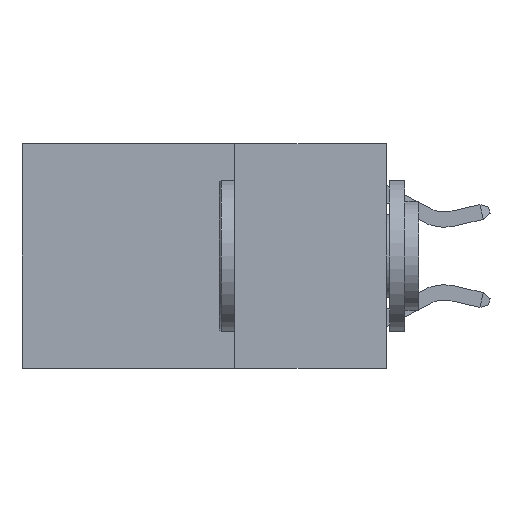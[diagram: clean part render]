
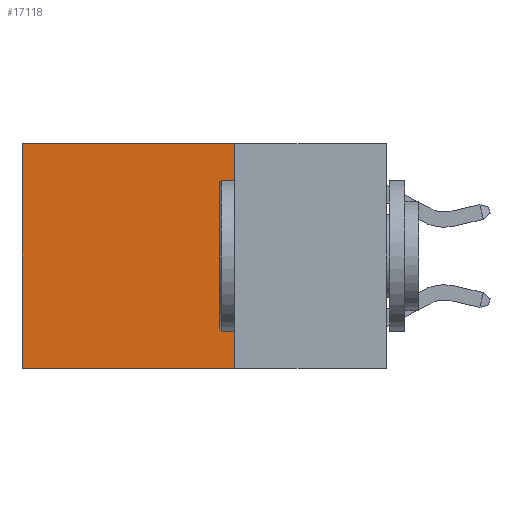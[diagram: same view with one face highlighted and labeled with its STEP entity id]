
A CAD part, left-side view. The second image highlights one B-rep face of the part: STEP entity #17118.
In plain terms, the highlighted planar face has unit normal (-1, 0, 0).
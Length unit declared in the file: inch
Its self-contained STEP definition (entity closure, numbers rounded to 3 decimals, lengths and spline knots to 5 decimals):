
#227 = FACE_OUTER_BOUND ( 'NONE', #14851, .T. ) ;
#1651 = CARTESIAN_POINT ( 'NONE',  ( 0.2625, 0.25, -0.37 ) ) ;
#2947 = CARTESIAN_POINT ( 'NONE',  ( 0.2625, 0.25, 0. ) ) ;
#3450 = EDGE_CURVE ( 'NONE', #28024, #12084, #20309, .T. ) ;
#3762 = CARTESIAN_POINT ( 'NONE',  ( 0.2625, 0.25, 0. ) ) ;
#4168 = DIRECTION ( 'NONE',  ( 0., 0., -1. ) ) ;
#4208 = DIRECTION ( 'NONE',  ( 0., 1., 0. ) ) ;
#4319 = LINE ( 'NONE', #11555, #26638 ) ;
#5220 = PLANE ( 'NONE',  #27787 ) ;
#6263 = EDGE_CURVE ( 'NONE', #12767, #10759, #6790, .T. ) ;
#6790 = LINE ( 'NONE', #1651, #8240 ) ;
#7896 = CARTESIAN_POINT ( 'NONE',  ( 0.2625, 0.6, -0.37 ) ) ;
#8240 = VECTOR ( 'NONE', #22434, 39.37008 ) ;
#9459 = DIRECTION ( 'NONE',  ( 1., 0., 0. ) ) ;
#9607 = DIRECTION ( 'NONE',  ( 0., 0., -1. ) ) ;
#10759 = VERTEX_POINT ( 'NONE', #7896 ) ;
#10929 = VECTOR ( 'NONE', #4208, 39.37008 ) ;
#11555 = CARTESIAN_POINT ( 'NONE',  ( 0.2625, 0.6, 0. ) ) ;
#12084 = VERTEX_POINT ( 'NONE', #19352 ) ;
#12743 = CARTESIAN_POINT ( 'NONE',  ( 0.2625, 0.25, 0. ) ) ;
#12767 = VERTEX_POINT ( 'NONE', #17375 ) ;
#12930 = CARTESIAN_POINT ( 'NONE',  ( 0.2625, 0.25, 0. ) ) ;
#14851 = EDGE_LOOP ( 'NONE', ( #19906, #29104, #19810, #22717 ) ) ;
#15357 = EDGE_CURVE ( 'NONE', #28024, #12767, #16848, .T. ) ;
#16848 = LINE ( 'NONE', #12930, #25808 ) ;
#17118 = ADVANCED_FACE ( 'NONE', ( #227 ), #5220, .F. ) ;
#17375 = CARTESIAN_POINT ( 'NONE',  ( 0.2625, 0.25, -0.37 ) ) ;
#19352 = CARTESIAN_POINT ( 'NONE',  ( 0.2625, 0.6, 0. ) ) ;
#19810 = ORIENTED_EDGE ( 'NONE', *, *, #15357, .F. ) ;
#19906 = ORIENTED_EDGE ( 'NONE', *, *, #21572, .T. ) ;
#20309 = LINE ( 'NONE', #3762, #10929 ) ;
#21572 = EDGE_CURVE ( 'NONE', #12084, #10759, #4319, .T. ) ;
#22099 = DIRECTION ( 'NONE',  ( 0., 0., -1. ) ) ;
#22434 = DIRECTION ( 'NONE',  ( 0., 1., 0. ) ) ;
#22717 = ORIENTED_EDGE ( 'NONE', *, *, #3450, .T. ) ;
#25808 = VECTOR ( 'NONE', #22099, 39.37008 ) ;
#26638 = VECTOR ( 'NONE', #4168, 39.37008 ) ;
#27787 = AXIS2_PLACEMENT_3D ( 'NONE', #2947, #9459, #9607 ) ;
#28024 = VERTEX_POINT ( 'NONE', #12743 ) ;
#29104 = ORIENTED_EDGE ( 'NONE', *, *, #6263, .F. ) ;
